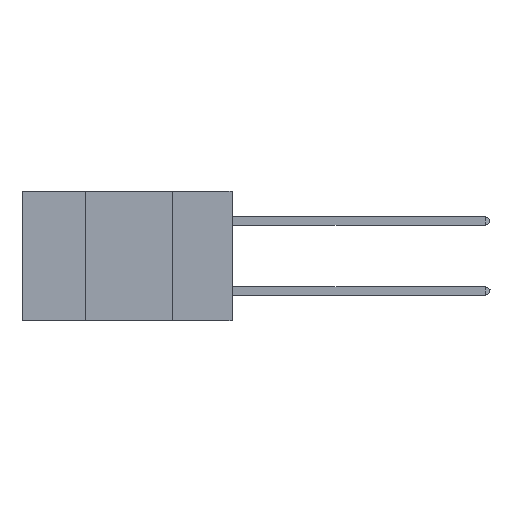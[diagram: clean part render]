
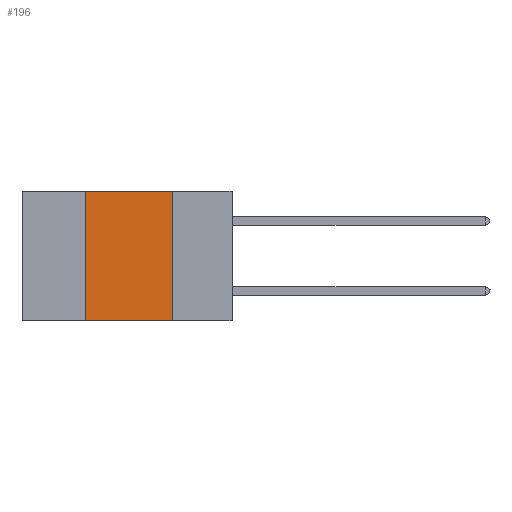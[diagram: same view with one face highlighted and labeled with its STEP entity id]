
A CAD part, left-side view. The second image highlights one B-rep face of the part: STEP entity #196.
In plain terms, the highlighted planar face has unit normal (-1, 0, 0).
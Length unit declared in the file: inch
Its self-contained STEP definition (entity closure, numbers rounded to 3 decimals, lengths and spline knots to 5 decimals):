
#196 = ADVANCED_FACE ( 'NONE', ( #15090 ), #3647, .F. ) ;
#235 = LINE ( 'NONE', #15700, #20362 ) ;
#463 = ORIENTED_EDGE ( 'NONE', *, *, #26779, .F. ) ;
#744 = EDGE_CURVE ( 'NONE', #13079, #3447, #26867, .T. ) ;
#2075 = ORIENTED_EDGE ( 'NONE', *, *, #6298, .F. ) ;
#2679 = DIRECTION ( 'NONE',  ( 0., 0., -1. ) ) ;
#3093 = CARTESIAN_POINT ( 'NONE',  ( 0., 0.42, 0. ) ) ;
#3420 = DIRECTION ( 'NONE',  ( 0., -1., 0. ) ) ;
#3447 = VERTEX_POINT ( 'NONE', #6573 ) ;
#3647 = PLANE ( 'NONE',  #18741 ) ;
#3777 = CARTESIAN_POINT ( 'NONE',  ( 0., 0.17, 0. ) ) ;
#3839 = DIRECTION ( 'NONE',  ( 0., 0., 1. ) ) ;
#4154 = CARTESIAN_POINT ( 'NONE',  ( 0., 0.6, -0.37 ) ) ;
#5809 = ORIENTED_EDGE ( 'NONE', *, *, #744, .T. ) ;
#6298 = EDGE_CURVE ( 'NONE', #8156, #3447, #235, .T. ) ;
#6573 = CARTESIAN_POINT ( 'NONE',  ( 0., 0.17, -0.37 ) ) ;
#7772 = DIRECTION ( 'NONE',  ( 0., 0., -1. ) ) ;
#8078 = VECTOR ( 'NONE', #15483, 39.37008 ) ;
#8156 = VERTEX_POINT ( 'NONE', #3777 ) ;
#9225 = VECTOR ( 'NONE', #3839, 39.37008 ) ;
#10973 = EDGE_LOOP ( 'NONE', ( #2075, #17367, #463, #5809 ) ) ;
#13079 = VERTEX_POINT ( 'NONE', #27197 ) ;
#13325 = VERTEX_POINT ( 'NONE', #3093 ) ;
#14488 = EDGE_CURVE ( 'NONE', #13325, #8156, #15868, .T. ) ;
#15090 = FACE_OUTER_BOUND ( 'NONE', #10973, .T. ) ;
#15483 = DIRECTION ( 'NONE',  ( 0., -1., 0. ) ) ;
#15700 = CARTESIAN_POINT ( 'NONE',  ( 0., 0.17, 0. ) ) ;
#15868 = LINE ( 'NONE', #16477, #18273 ) ;
#16477 = CARTESIAN_POINT ( 'NONE',  ( 0., 0.6, 0. ) ) ;
#17367 = ORIENTED_EDGE ( 'NONE', *, *, #14488, .F. ) ;
#18273 = VECTOR ( 'NONE', #3420, 39.37008 ) ;
#18741 = AXIS2_PLACEMENT_3D ( 'NONE', #20698, #25109, #7772 ) ;
#20362 = VECTOR ( 'NONE', #2679, 39.37008 ) ;
#20698 = CARTESIAN_POINT ( 'NONE',  ( 0., 0.6, 0. ) ) ;
#22192 = LINE ( 'NONE', #25565, #9225 ) ;
#25109 = DIRECTION ( 'NONE',  ( 1., 0., 0. ) ) ;
#25565 = CARTESIAN_POINT ( 'NONE',  ( 0., 0.42, 0. ) ) ;
#26779 = EDGE_CURVE ( 'NONE', #13079, #13325, #22192, .T. ) ;
#26867 = LINE ( 'NONE', #4154, #8078 ) ;
#27197 = CARTESIAN_POINT ( 'NONE',  ( 0., 0.42, -0.37 ) ) ;
